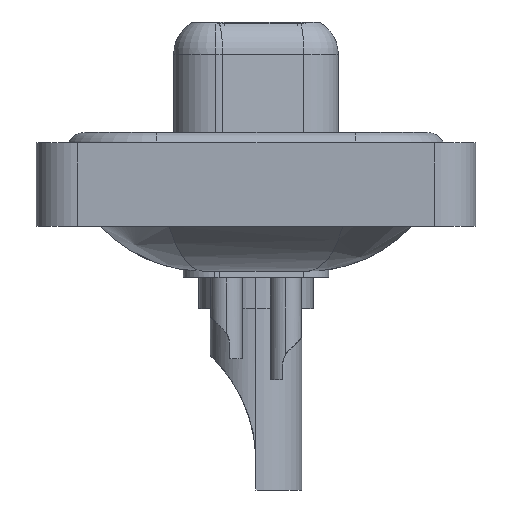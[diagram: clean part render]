
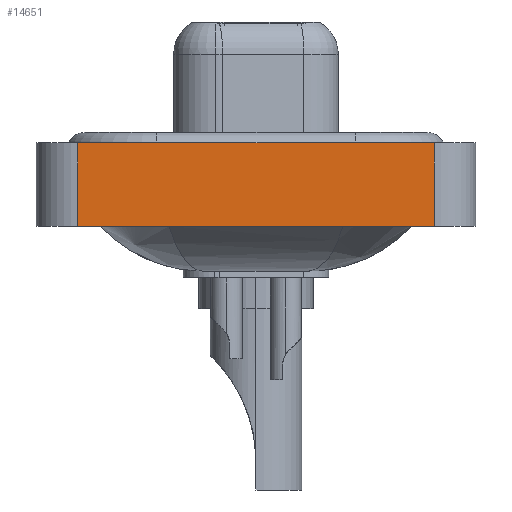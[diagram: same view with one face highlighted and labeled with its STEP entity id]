
A CAD part, left-side view. The second image highlights one B-rep face of the part: STEP entity #14651.
In plain terms, the highlighted planar face has unit normal (-1, 0, 0).
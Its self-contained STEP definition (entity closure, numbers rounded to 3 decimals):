
#527 = VECTOR ( 'NONE', #18846, 1000. ) ;
#784 = EDGE_CURVE ( 'NONE', #13605, #3432, #12048, .T. ) ;
#1568 = DIRECTION ( 'NONE',  ( 0., -1., 0. ) ) ;
#2227 = LINE ( 'NONE', #5901, #12811 ) ;
#2297 = EDGE_CURVE ( 'NONE', #13605, #17689, #21319, .T. ) ;
#2839 = EDGE_CURVE ( 'NONE', #17689, #8322, #2227, .T. ) ;
#2838 = VECTOR ( 'NONE', #14539, 1000. ) ;
#3432 = VERTEX_POINT ( 'NONE', #4583 ) ;
#4583 = CARTESIAN_POINT ( 'NONE',  ( -7.3, 8.55, 0.4 ) ) ;
#4736 = DIRECTION ( 'NONE',  ( 0., 0., 1. ) ) ;
#5901 = CARTESIAN_POINT ( 'NONE',  ( -7.3, -8.55, -3.6 ) ) ;
#6481 = PLANE ( 'NONE',  #21803 ) ;
#6541 = VECTOR ( 'NONE', #1568, 1000. ) ;
#6762 = ORIENTED_EDGE ( 'NONE', *, *, #2297, .T. ) ;
#7536 = CARTESIAN_POINT ( 'NONE',  ( -7.3, -8.55, -3.6 ) ) ;
#8317 = CARTESIAN_POINT ( 'NONE',  ( -7.3, -8.55, -3.6 ) ) ;
#8322 = VERTEX_POINT ( 'NONE', #16972 ) ;
#10150 = EDGE_CURVE ( 'NONE', #3432, #8322, #15240, .T. ) ;
#10215 = CARTESIAN_POINT ( 'NONE',  ( -7.3, 8.55, -3.6 ) ) ;
#10583 = CARTESIAN_POINT ( 'NONE',  ( -7.3, 8.55, -3.6 ) ) ;
#10716 = DIRECTION ( 'NONE',  ( 0., 0., 1. ) ) ;
#10856 = EDGE_LOOP ( 'NONE', ( #17747, #15204, #20388, #6762 ) ) ;
#12048 = LINE ( 'NONE', #10215, #527 ) ;
#12811 = VECTOR ( 'NONE', #10716, 1000. ) ;
#13605 = VERTEX_POINT ( 'NONE', #10583 ) ;
#14539 = DIRECTION ( 'NONE',  ( 0., -1., 0. ) ) ;
#14651 = ADVANCED_FACE ( 'NONE', ( #20266 ), #6481, .T. ) ;
#14968 = DIRECTION ( 'NONE',  ( -1., 0., 0. ) ) ;
#15204 = ORIENTED_EDGE ( 'NONE', *, *, #10150, .F. ) ;
#15240 = LINE ( 'NONE', #22699, #6541 ) ;
#16972 = CARTESIAN_POINT ( 'NONE',  ( -7.3, -8.55, 0.4 ) ) ;
#17689 = VERTEX_POINT ( 'NONE', #21022 ) ;
#17747 = ORIENTED_EDGE ( 'NONE', *, *, #2839, .T. ) ;
#18846 = DIRECTION ( 'NONE',  ( 0., 0., 1. ) ) ;
#20266 = FACE_OUTER_BOUND ( 'NONE', #10856, .T. ) ;
#20388 = ORIENTED_EDGE ( 'NONE', *, *, #784, .F. ) ;
#21022 = CARTESIAN_POINT ( 'NONE',  ( -7.3, -8.55, -3.6 ) ) ;
#21319 = LINE ( 'NONE', #7536, #2838 ) ;
#21803 = AXIS2_PLACEMENT_3D ( 'NONE', #8317, #14968, #4736 ) ;
#22699 = CARTESIAN_POINT ( 'NONE',  ( -7.3, -8.55, 0.4 ) ) ;
